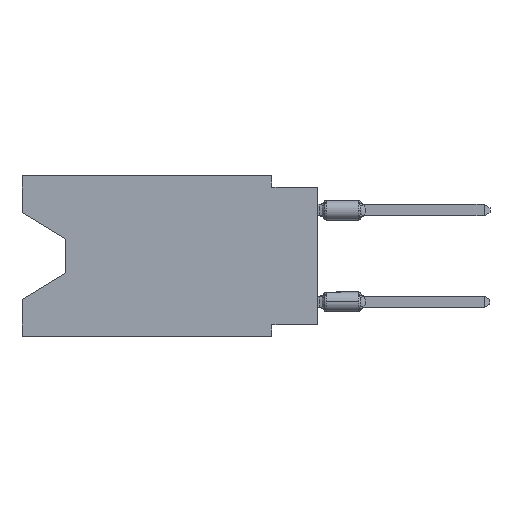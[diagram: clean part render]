
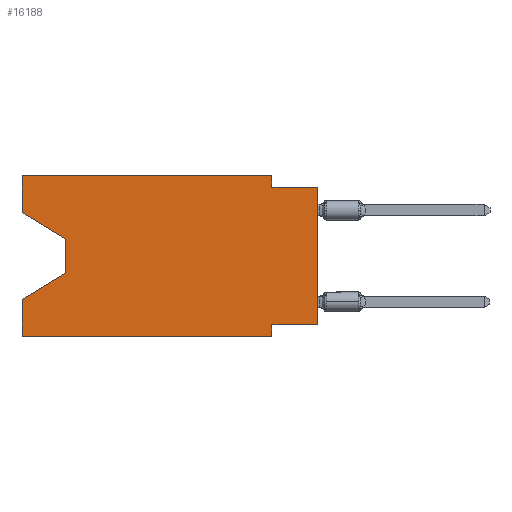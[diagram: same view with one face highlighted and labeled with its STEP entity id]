
A CAD part, left-side view. The second image highlights one B-rep face of the part: STEP entity #16188.
In plain terms, the highlighted planar face has unit normal (-1, 0, 0).
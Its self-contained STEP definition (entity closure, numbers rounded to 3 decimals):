
#9 = LINE ( 'NONE', #8402, #7393 ) ;
#40 = ORIENTED_EDGE ( 'NONE', *, *, #11396, .F. ) ;
#327 = ORIENTED_EDGE ( 'NONE', *, *, #11987, .T. ) ;
#376 = EDGE_CURVE ( 'NONE', #8910, #2385, #15161, .T. ) ;
#454 = VECTOR ( 'NONE', #8144, 1000. ) ;
#873 = VECTOR ( 'NONE', #3223, 1000. ) ;
#917 = VECTOR ( 'NONE', #6543, 1000. ) ;
#1019 = VERTEX_POINT ( 'NONE', #5727 ) ;
#1705 = DIRECTION ( 'NONE',  ( 1., 0., 0. ) ) ;
#1982 = EDGE_CURVE ( 'NONE', #16415, #20990, #14971, .T. ) ;
#2150 = CARTESIAN_POINT ( 'NONE',  ( 0., 2.54, -8.89 ) ) ;
#2319 = VERTEX_POINT ( 'NONE', #7690 ) ;
#2334 = ORIENTED_EDGE ( 'NONE', *, *, #12168, .F. ) ;
#2385 = VERTEX_POINT ( 'NONE', #13305 ) ;
#2725 = DIRECTION ( 'NONE',  ( 0., 0., 1. ) ) ;
#3125 = VECTOR ( 'NONE', #16959, 1000. ) ;
#3223 = DIRECTION ( 'NONE',  ( 0., 0., -1. ) ) ;
#3295 = DIRECTION ( 'NONE',  ( 0., 0., -1. ) ) ;
#3601 = EDGE_CURVE ( 'NONE', #8910, #9262, #18756, .T. ) ;
#4447 = VECTOR ( 'NONE', #21763, 1000. ) ;
#4625 = VERTEX_POINT ( 'NONE', #19858 ) ;
#5074 = CARTESIAN_POINT ( 'NONE',  ( 0., 16.383, 0. ) ) ;
#5518 = VECTOR ( 'NONE', #13668, 1000. ) ;
#5727 = CARTESIAN_POINT ( 'NONE',  ( 0., 0., -8.255 ) ) ;
#6543 = DIRECTION ( 'NONE',  ( 0., 0.855, -0.519 ) ) ;
#6584 = VECTOR ( 'NONE', #3295, 1000. ) ;
#6741 = LINE ( 'NONE', #19139, #454 ) ;
#6828 = PLANE ( 'NONE',  #20959 ) ;
#7099 = EDGE_CURVE ( 'NONE', #16415, #8228, #10289, .T. ) ;
#7121 = ORIENTED_EDGE ( 'NONE', *, *, #7099, .F. ) ;
#7222 = CARTESIAN_POINT ( 'NONE',  ( 0., 13.97, -5.385 ) ) ;
#7393 = VECTOR ( 'NONE', #12371, 1000. ) ;
#7690 = CARTESIAN_POINT ( 'NONE',  ( 0., 2.54, -0.635 ) ) ;
#8060 = LINE ( 'NONE', #9691, #5518 ) ;
#8062 = CARTESIAN_POINT ( 'NONE',  ( 0., 13.97, -5.385 ) ) ;
#8144 = DIRECTION ( 'NONE',  ( 0., 0., -1. ) ) ;
#8228 = VERTEX_POINT ( 'NONE', #10084 ) ;
#8402 = CARTESIAN_POINT ( 'NONE',  ( 0., 0., -0.635 ) ) ;
#8821 = DIRECTION ( 'NONE',  ( 0., 0., -1. ) ) ;
#8827 = CARTESIAN_POINT ( 'NONE',  ( 0., 16.383, -2.038 ) ) ;
#8910 = VERTEX_POINT ( 'NONE', #8827 ) ;
#9101 = VERTEX_POINT ( 'NONE', #7222 ) ;
#9262 = VERTEX_POINT ( 'NONE', #16467 ) ;
#9691 = CARTESIAN_POINT ( 'NONE',  ( 0., 0., 0. ) ) ;
#9796 = ORIENTED_EDGE ( 'NONE', *, *, #3601, .F. ) ;
#9922 = VECTOR ( 'NONE', #20056, 1000. ) ;
#9951 = VECTOR ( 'NONE', #18569, 1000. ) ;
#9982 = ORIENTED_EDGE ( 'NONE', *, *, #17985, .T. ) ;
#10084 = CARTESIAN_POINT ( 'NONE',  ( 0., 16.383, -6.852 ) ) ;
#10182 = CARTESIAN_POINT ( 'NONE',  ( 0., 16.383, 0. ) ) ;
#10289 = LINE ( 'NONE', #22003, #4447 ) ;
#10455 = FACE_OUTER_BOUND ( 'NONE', #12218, .T. ) ;
#10499 = EDGE_CURVE ( 'NONE', #2385, #9101, #21423, .T. ) ;
#11212 = ORIENTED_EDGE ( 'NONE', *, *, #20189, .F. ) ;
#11258 = LINE ( 'NONE', #16781, #9922 ) ;
#11396 = EDGE_CURVE ( 'NONE', #9262, #16451, #21108, .T. ) ;
#11800 = CARTESIAN_POINT ( 'NONE',  ( 0., 0., -0.635 ) ) ;
#11987 = EDGE_CURVE ( 'NONE', #1019, #19193, #8060, .T. ) ;
#12168 = EDGE_CURVE ( 'NONE', #2319, #19193, #9, .T. ) ;
#12218 = EDGE_LOOP ( 'NONE', ( #20430, #18099, #9982, #7121, #21828, #11212, #15230, #327, #2334, #21215, #40, #9796 ) ) ;
#12371 = DIRECTION ( 'NONE',  ( 0., -1., 0. ) ) ;
#13305 = CARTESIAN_POINT ( 'NONE',  ( 0., 13.97, -3.505 ) ) ;
#13553 = CARTESIAN_POINT ( 'NONE',  ( 0., 16.383, -8.89 ) ) ;
#13668 = DIRECTION ( 'NONE',  ( 0., 0., 1. ) ) ;
#14643 = LINE ( 'NONE', #2150, #873 ) ;
#14971 = LINE ( 'NONE', #18829, #3125 ) ;
#15161 = LINE ( 'NONE', #20439, #9951 ) ;
#15230 = ORIENTED_EDGE ( 'NONE', *, *, #17334, .F. ) ;
#15423 = LINE ( 'NONE', #8062, #917 ) ;
#15831 = DIRECTION ( 'NONE',  ( 0., -1., 0. ) ) ;
#16188 = ADVANCED_FACE ( 'NONE', ( #10455 ), #6828, .F. ) ;
#16415 = VERTEX_POINT ( 'NONE', #13553 ) ;
#16451 = VERTEX_POINT ( 'NONE', #21059 ) ;
#16467 = CARTESIAN_POINT ( 'NONE',  ( 0., 16.383, 0. ) ) ;
#16648 = EDGE_CURVE ( 'NONE', #16451, #2319, #6741, .T. ) ;
#16781 = CARTESIAN_POINT ( 'NONE',  ( 0., 0., -8.255 ) ) ;
#16920 = CARTESIAN_POINT ( 'NONE',  ( 0., 2.54, -8.89 ) ) ;
#16959 = DIRECTION ( 'NONE',  ( 0., -1., 0. ) ) ;
#17334 = EDGE_CURVE ( 'NONE', #1019, #4625, #11258, .T. ) ;
#17730 = CARTESIAN_POINT ( 'NONE',  ( 0., 16.383, 0. ) ) ;
#17985 = EDGE_CURVE ( 'NONE', #9101, #8228, #15423, .T. ) ;
#18099 = ORIENTED_EDGE ( 'NONE', *, *, #10499, .T. ) ;
#18569 = DIRECTION ( 'NONE',  ( 0., -0.855, -0.519 ) ) ;
#18578 = VECTOR ( 'NONE', #15831, 1000. ) ;
#18756 = LINE ( 'NONE', #10182, #18803 ) ;
#18803 = VECTOR ( 'NONE', #2725, 1000. ) ;
#18829 = CARTESIAN_POINT ( 'NONE',  ( 0., 16.383, -8.89 ) ) ;
#19139 = CARTESIAN_POINT ( 'NONE',  ( 0., 2.54, 0. ) ) ;
#19193 = VERTEX_POINT ( 'NONE', #11800 ) ;
#19194 = CARTESIAN_POINT ( 'NONE',  ( 0., 13.97, -3.505 ) ) ;
#19858 = CARTESIAN_POINT ( 'NONE',  ( 0., 2.54, -8.255 ) ) ;
#20056 = DIRECTION ( 'NONE',  ( 0., 1., 0. ) ) ;
#20189 = EDGE_CURVE ( 'NONE', #4625, #20990, #14643, .T. ) ;
#20430 = ORIENTED_EDGE ( 'NONE', *, *, #376, .T. ) ;
#20439 = CARTESIAN_POINT ( 'NONE',  ( 0., 16.383, -2.038 ) ) ;
#20959 = AXIS2_PLACEMENT_3D ( 'NONE', #17730, #1705, #8821 ) ;
#20990 = VERTEX_POINT ( 'NONE', #16920 ) ;
#21059 = CARTESIAN_POINT ( 'NONE',  ( 0., 2.54, 0. ) ) ;
#21108 = LINE ( 'NONE', #5074, #18578 ) ;
#21215 = ORIENTED_EDGE ( 'NONE', *, *, #16648, .F. ) ;
#21423 = LINE ( 'NONE', #19194, #6584 ) ;
#21763 = DIRECTION ( 'NONE',  ( 0., 0., 1. ) ) ;
#21828 = ORIENTED_EDGE ( 'NONE', *, *, #1982, .T. ) ;
#22003 = CARTESIAN_POINT ( 'NONE',  ( 0., 16.383, 0. ) ) ;
